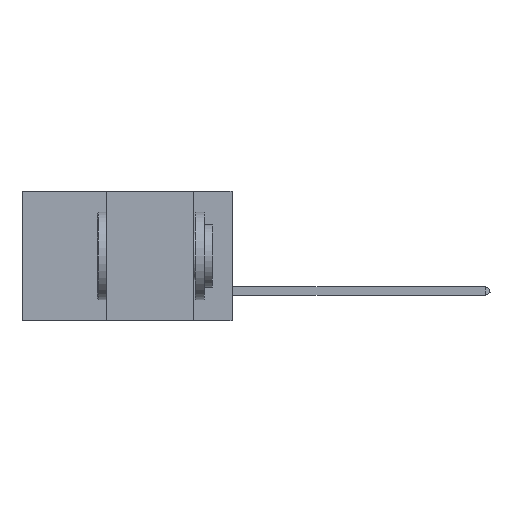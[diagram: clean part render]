
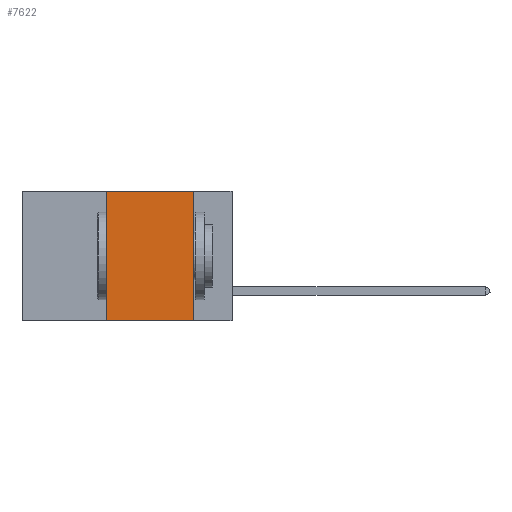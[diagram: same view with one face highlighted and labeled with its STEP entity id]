
A CAD part, left-side view. The second image highlights one B-rep face of the part: STEP entity #7622.
In plain terms, the highlighted planar face has unit normal (-1, 0, 0).
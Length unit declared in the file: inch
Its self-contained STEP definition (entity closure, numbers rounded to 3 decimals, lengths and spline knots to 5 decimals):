
#472 = EDGE_CURVE ( 'NONE', #4821, #2673, #3412, .T. ) ;
#860 = DIRECTION ( 'NONE',  ( 0., -1., 0. ) ) ;
#935 = EDGE_CURVE ( 'NONE', #8004, #2673, #2838, .T. ) ;
#1085 = DIRECTION ( 'NONE',  ( 0., 0., 1. ) ) ;
#1295 = CARTESIAN_POINT ( 'NONE',  ( 0., 0.11, 0. ) ) ;
#1537 = DIRECTION ( 'NONE',  ( 0., -1., 0. ) ) ;
#2383 = ORIENTED_EDGE ( 'NONE', *, *, #935, .F. ) ;
#2673 = VERTEX_POINT ( 'NONE', #7244 ) ;
#2738 = CARTESIAN_POINT ( 'NONE',  ( 0., 0.36, 0. ) ) ;
#2838 = LINE ( 'NONE', #1295, #6112 ) ;
#2963 = DIRECTION ( 'NONE',  ( 1., 0., 0. ) ) ;
#3025 = CARTESIAN_POINT ( 'NONE',  ( 0., 0.6, -0.37 ) ) ;
#3412 = LINE ( 'NONE', #3025, #6919 ) ;
#3568 = ORIENTED_EDGE ( 'NONE', *, *, #8920, .F. ) ;
#3611 = DIRECTION ( 'NONE',  ( 0., 0., -1. ) ) ;
#4182 = CARTESIAN_POINT ( 'NONE',  ( 0., 0.6, 0. ) ) ;
#4270 = DIRECTION ( 'NONE',  ( 0., 0., -1. ) ) ;
#4821 = VERTEX_POINT ( 'NONE', #6413 ) ;
#5771 = ORIENTED_EDGE ( 'NONE', *, *, #8808, .F. ) ;
#5936 = CARTESIAN_POINT ( 'NONE',  ( 0., 0.6, 0. ) ) ;
#6052 = CARTESIAN_POINT ( 'NONE',  ( 0., 0.11, 0. ) ) ;
#6112 = VECTOR ( 'NONE', #4270, 39.37008 ) ;
#6256 = CARTESIAN_POINT ( 'NONE',  ( 0., 0.36, 0. ) ) ;
#6316 = VECTOR ( 'NONE', #1085, 39.37008 ) ;
#6413 = CARTESIAN_POINT ( 'NONE',  ( 0., 0.36, -0.37 ) ) ;
#6428 = LINE ( 'NONE', #5936, #9067 ) ;
#6919 = VECTOR ( 'NONE', #860, 39.37008 ) ;
#7184 = EDGE_LOOP ( 'NONE', ( #2383, #5771, #3568, #9460 ) ) ;
#7244 = CARTESIAN_POINT ( 'NONE',  ( 0., 0.11, -0.37 ) ) ;
#7622 = ADVANCED_FACE ( 'NONE', ( #8758 ), #7947, .F. ) ;
#7667 = AXIS2_PLACEMENT_3D ( 'NONE', #4182, #2963, #3611 ) ;
#7947 = PLANE ( 'NONE',  #7667 ) ;
#8004 = VERTEX_POINT ( 'NONE', #6052 ) ;
#8279 = LINE ( 'NONE', #6256, #6316 ) ;
#8468 = VERTEX_POINT ( 'NONE', #2738 ) ;
#8758 = FACE_OUTER_BOUND ( 'NONE', #7184, .T. ) ;
#8808 = EDGE_CURVE ( 'NONE', #8468, #8004, #6428, .T. ) ;
#8920 = EDGE_CURVE ( 'NONE', #4821, #8468, #8279, .T. ) ;
#9067 = VECTOR ( 'NONE', #1537, 39.37008 ) ;
#9460 = ORIENTED_EDGE ( 'NONE', *, *, #472, .T. ) ;
